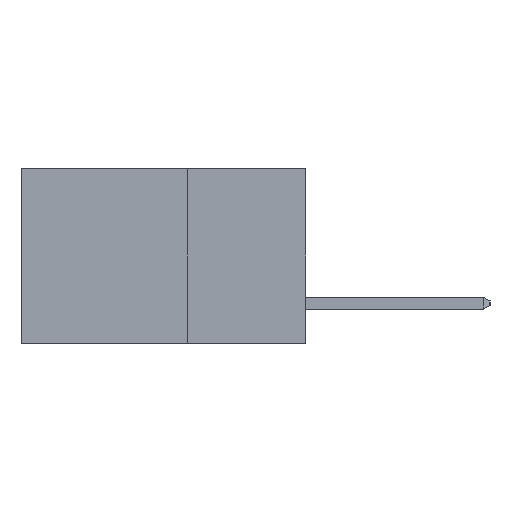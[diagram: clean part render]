
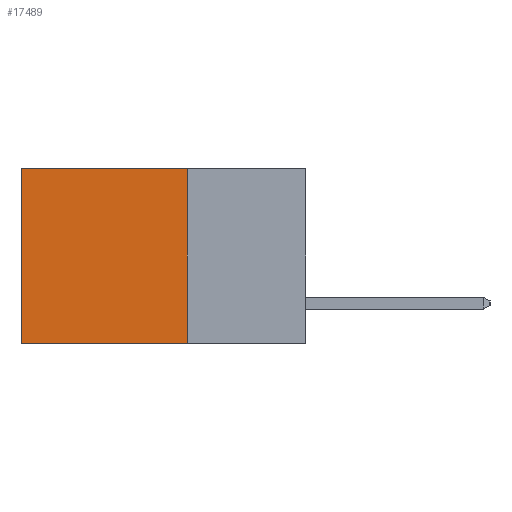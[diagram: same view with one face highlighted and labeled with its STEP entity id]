
A CAD part, left-side view. The second image highlights one B-rep face of the part: STEP entity #17489.
In plain terms, the highlighted planar face has unit normal (-1, 0, 0).
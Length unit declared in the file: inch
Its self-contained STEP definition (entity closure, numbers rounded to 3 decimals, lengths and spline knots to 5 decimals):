
#1064 = DIRECTION ( 'NONE',  ( 0., 1., 0. ) ) ;
#1392 = EDGE_CURVE ( 'NONE', #24204, #2620, #2800, .T. ) ;
#1399 = CARTESIAN_POINT ( 'NONE',  ( 0.298, 0.25, 0. ) ) ;
#2619 = VECTOR ( 'NONE', #6435, 39.37008 ) ;
#2620 = VERTEX_POINT ( 'NONE', #3641 ) ;
#2694 = VECTOR ( 'NONE', #4424, 39.37008 ) ;
#2800 = LINE ( 'NONE', #21550, #24440 ) ;
#3641 = CARTESIAN_POINT ( 'NONE',  ( 0.298, 0.6, -0.37 ) ) ;
#3963 = PLANE ( 'NONE',  #18619 ) ;
#4424 = DIRECTION ( 'NONE',  ( 0., 0., -1. ) ) ;
#5259 = ORIENTED_EDGE ( 'NONE', *, *, #9990, .F. ) ;
#5364 = LINE ( 'NONE', #1399, #11678 ) ;
#5422 = CARTESIAN_POINT ( 'NONE',  ( 0.298, 0.25, 0. ) ) ;
#5775 = DIRECTION ( 'NONE',  ( 0., 0., -1. ) ) ;
#6123 = CARTESIAN_POINT ( 'NONE',  ( 0.298, 0.25, -0.37 ) ) ;
#6238 = ORIENTED_EDGE ( 'NONE', *, *, #13133, .T. ) ;
#6435 = DIRECTION ( 'NONE',  ( 0., 1., 0. ) ) ;
#6913 = ORIENTED_EDGE ( 'NONE', *, *, #1392, .T. ) ;
#8212 = DIRECTION ( 'NONE',  ( 0., 0., -1. ) ) ;
#8222 = LINE ( 'NONE', #6123, #2619 ) ;
#8711 = EDGE_CURVE ( 'NONE', #20698, #11421, #13916, .T. ) ;
#8808 = EDGE_LOOP ( 'NONE', ( #6913, #5259, #23813, #6238 ) ) ;
#9990 = EDGE_CURVE ( 'NONE', #11421, #2620, #8222, .T. ) ;
#10891 = CARTESIAN_POINT ( 'NONE',  ( 0.298, 0.6, 0. ) ) ;
#11421 = VERTEX_POINT ( 'NONE', #19275 ) ;
#11678 = VECTOR ( 'NONE', #1064, 39.37008 ) ;
#13133 = EDGE_CURVE ( 'NONE', #20698, #24204, #5364, .T. ) ;
#13649 = FACE_OUTER_BOUND ( 'NONE', #8808, .T. ) ;
#13916 = LINE ( 'NONE', #5422, #2694 ) ;
#17205 = CARTESIAN_POINT ( 'NONE',  ( 0.298, 0.25, 0. ) ) ;
#17489 = ADVANCED_FACE ( 'NONE', ( #13649 ), #3963, .F. ) ;
#18619 = AXIS2_PLACEMENT_3D ( 'NONE', #18681, #20771, #8212 ) ;
#18681 = CARTESIAN_POINT ( 'NONE',  ( 0.298, 0.25, 0. ) ) ;
#19275 = CARTESIAN_POINT ( 'NONE',  ( 0.298, 0.25, -0.37 ) ) ;
#20698 = VERTEX_POINT ( 'NONE', #17205 ) ;
#20771 = DIRECTION ( 'NONE',  ( 1., 0., 0. ) ) ;
#21550 = CARTESIAN_POINT ( 'NONE',  ( 0.298, 0.6, 0. ) ) ;
#23813 = ORIENTED_EDGE ( 'NONE', *, *, #8711, .F. ) ;
#24204 = VERTEX_POINT ( 'NONE', #10891 ) ;
#24440 = VECTOR ( 'NONE', #5775, 39.37008 ) ;
